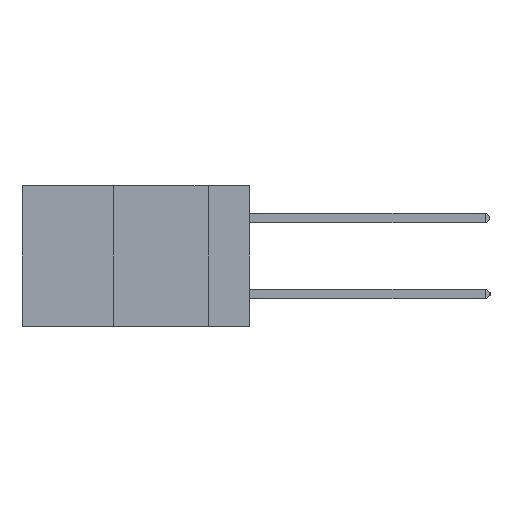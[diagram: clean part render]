
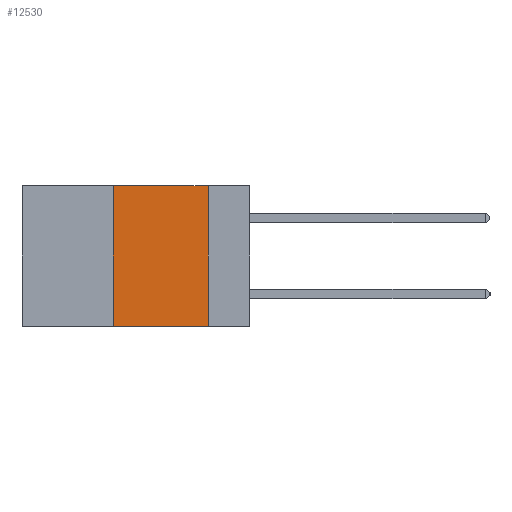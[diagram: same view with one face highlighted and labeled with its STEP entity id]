
A CAD part, left-side view. The second image highlights one B-rep face of the part: STEP entity #12530.
In plain terms, the highlighted planar face has unit normal (-1, 0, 0).
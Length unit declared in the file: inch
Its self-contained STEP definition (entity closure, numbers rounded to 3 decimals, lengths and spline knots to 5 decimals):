
#59 = ORIENTED_EDGE ( 'NONE', *, *, #24484, .F. ) ;
#216 = CARTESIAN_POINT ( 'NONE',  ( 0., 0.36, -0.37 ) ) ;
#1177 = FACE_OUTER_BOUND ( 'NONE', #16881, .T. ) ;
#2218 = VECTOR ( 'NONE', #17345, 39.37008 ) ;
#2630 = DIRECTION ( 'NONE',  ( 0., -1., 0. ) ) ;
#2781 = VERTEX_POINT ( 'NONE', #216 ) ;
#2998 = CARTESIAN_POINT ( 'NONE',  ( 0., 0.11, -0.37 ) ) ;
#3533 = VECTOR ( 'NONE', #11138, 39.37008 ) ;
#3798 = PLANE ( 'NONE',  #12900 ) ;
#5019 = CARTESIAN_POINT ( 'NONE',  ( 0., 0.36, 0. ) ) ;
#7293 = CARTESIAN_POINT ( 'NONE',  ( 0., 0.6, -0.37 ) ) ;
#8341 = VECTOR ( 'NONE', #15127, 39.37008 ) ;
#8750 = VERTEX_POINT ( 'NONE', #2998 ) ;
#9411 = DIRECTION ( 'NONE',  ( 0., 0., -1. ) ) ;
#9545 = LINE ( 'NONE', #14114, #21518 ) ;
#9792 = EDGE_CURVE ( 'NONE', #2781, #21716, #19238, .T. ) ;
#10102 = ORIENTED_EDGE ( 'NONE', *, *, #22457, .T. ) ;
#10860 = CARTESIAN_POINT ( 'NONE',  ( 0., 0.11, 0. ) ) ;
#11138 = DIRECTION ( 'NONE',  ( 0., 0., -1. ) ) ;
#11299 = CARTESIAN_POINT ( 'NONE',  ( 0., 0.6, 0. ) ) ;
#12530 = ADVANCED_FACE ( 'NONE', ( #1177 ), #3798, .F. ) ;
#12900 = AXIS2_PLACEMENT_3D ( 'NONE', #11299, #13292, #9411 ) ;
#13292 = DIRECTION ( 'NONE',  ( 1., 0., 0. ) ) ;
#13636 = VERTEX_POINT ( 'NONE', #10860 ) ;
#14114 = CARTESIAN_POINT ( 'NONE',  ( 0., 0.6, 0. ) ) ;
#15127 = DIRECTION ( 'NONE',  ( 0., -1., 0. ) ) ;
#15600 = CARTESIAN_POINT ( 'NONE',  ( 0., 0.36, 0. ) ) ;
#16219 = ORIENTED_EDGE ( 'NONE', *, *, #19753, .F. ) ;
#16881 = EDGE_LOOP ( 'NONE', ( #16219, #59, #19956, #10102 ) ) ;
#17345 = DIRECTION ( 'NONE',  ( 0., 0., 1. ) ) ;
#19183 = LINE ( 'NONE', #7293, #8341 ) ;
#19238 = LINE ( 'NONE', #15600, #2218 ) ;
#19753 = EDGE_CURVE ( 'NONE', #13636, #8750, #21700, .T. ) ;
#19956 = ORIENTED_EDGE ( 'NONE', *, *, #9792, .F. ) ;
#21518 = VECTOR ( 'NONE', #2630, 39.37008 ) ;
#21700 = LINE ( 'NONE', #22633, #3533 ) ;
#21716 = VERTEX_POINT ( 'NONE', #5019 ) ;
#22457 = EDGE_CURVE ( 'NONE', #2781, #8750, #19183, .T. ) ;
#22633 = CARTESIAN_POINT ( 'NONE',  ( 0., 0.11, 0. ) ) ;
#24484 = EDGE_CURVE ( 'NONE', #21716, #13636, #9545, .T. ) ;
